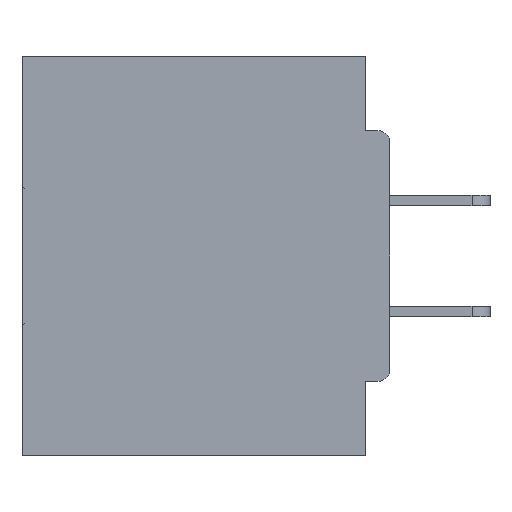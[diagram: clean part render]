
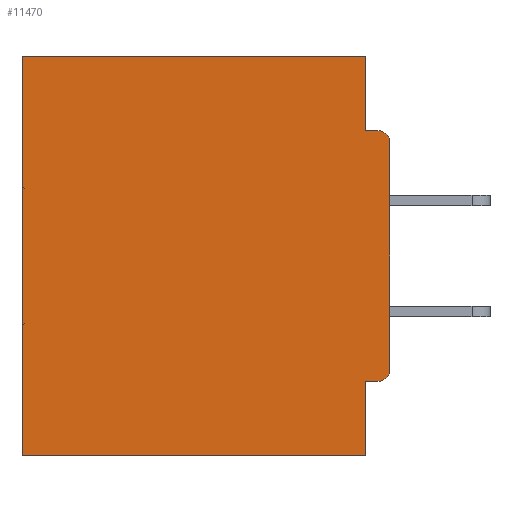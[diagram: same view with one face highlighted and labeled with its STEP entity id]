
A CAD part, left-side view. The second image highlights one B-rep face of the part: STEP entity #11470.
In plain terms, the highlighted planar face has unit normal (-1, 0, 0).
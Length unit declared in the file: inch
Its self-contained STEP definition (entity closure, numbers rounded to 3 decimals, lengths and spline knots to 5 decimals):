
#1285 = LINE ( 'NONE', #10455, #16708 ) ;
#1832 = VECTOR ( 'NONE', #39728, 39.37008 ) ;
#2207 = VERTEX_POINT ( 'NONE', #20075 ) ;
#2713 = LINE ( 'NONE', #6771, #37363 ) ;
#2864 = DIRECTION ( 'NONE',  ( -1., 0., 0. ) ) ;
#3424 = DIRECTION ( 'NONE',  ( 0., 0., -1. ) ) ;
#3531 = VERTEX_POINT ( 'NONE', #36057 ) ;
#3902 = VECTOR ( 'NONE', #17438, 39.37008 ) ;
#3994 = VECTOR ( 'NONE', #11558, 39.37008 ) ;
#5198 = ORIENTED_EDGE ( 'NONE', *, *, #39900, .T. ) ;
#5393 = CARTESIAN_POINT ( 'NONE',  ( 0.298, 0., -0.5 ) ) ;
#5711 = VERTEX_POINT ( 'NONE', #43050 ) ;
#5946 = CARTESIAN_POINT ( 'NONE',  ( 0.298, 0.46, 0. ) ) ;
#6062 = LINE ( 'NONE', #5393, #1832 ) ;
#6728 = EDGE_CURVE ( 'NONE', #20890, #8787, #16250, .T. ) ;
#6771 = CARTESIAN_POINT ( 'NONE',  ( 0.298, 0., -0.4065 ) ) ;
#6812 = VERTEX_POINT ( 'NONE', #8555 ) ;
#7296 = ORIENTED_EDGE ( 'NONE', *, *, #17299, .F. ) ;
#7655 = ORIENTED_EDGE ( 'NONE', *, *, #6728, .T. ) ;
#7831 = CARTESIAN_POINT ( 'NONE',  ( 0.298, 0., 0. ) ) ;
#8555 = CARTESIAN_POINT ( 'NONE',  ( 0.298, 0.46, -0.5 ) ) ;
#8787 = VERTEX_POINT ( 'NONE', #5946 ) ;
#10455 = CARTESIAN_POINT ( 'NONE',  ( 0.298, 0.031, -0.5 ) ) ;
#10601 = CIRCLE ( 'NONE', #30899, 0.015 ) ;
#10845 = ORIENTED_EDGE ( 'NONE', *, *, #43947, .F. ) ;
#11470 = ADVANCED_FACE ( 'NONE', ( #34854 ), #23864, .F. ) ;
#11558 = DIRECTION ( 'NONE',  ( 0., 1., 0. ) ) ;
#11743 = LINE ( 'NONE', #23046, #12156 ) ;
#12156 = VECTOR ( 'NONE', #16825, 39.37008 ) ;
#12641 = ORIENTED_EDGE ( 'NONE', *, *, #33715, .T. ) ;
#13978 = ORIENTED_EDGE ( 'NONE', *, *, #35095, .F. ) ;
#14409 = DIRECTION ( 'NONE',  ( 0., 0., -1. ) ) ;
#16011 = DIRECTION ( 'NONE',  ( 0., 0., -1. ) ) ;
#16181 = ORIENTED_EDGE ( 'NONE', *, *, #34183, .F. ) ;
#16250 = LINE ( 'NONE', #7831, #3994 ) ;
#16550 = VERTEX_POINT ( 'NONE', #39264 ) ;
#16708 = VECTOR ( 'NONE', #37703, 39.37008 ) ;
#16825 = DIRECTION ( 'NONE',  ( 0., 0., -1. ) ) ;
#17299 = EDGE_CURVE ( 'NONE', #5711, #6812, #6062, .T. ) ;
#17438 = DIRECTION ( 'NONE',  ( 0., -1., 0. ) ) ;
#18301 = CARTESIAN_POINT ( 'NONE',  ( 0.298, 0., -0.1085 ) ) ;
#19709 = AXIS2_PLACEMENT_3D ( 'NONE', #39305, #28441, #30352 ) ;
#20075 = CARTESIAN_POINT ( 'NONE',  ( 0.298, 0., -0.3915 ) ) ;
#20427 = CARTESIAN_POINT ( 'NONE',  ( 0.298, 0.031, -0.0935 ) ) ;
#20545 = EDGE_LOOP ( 'NONE', ( #12641, #37215, #16181, #7655, #5198, #7296, #10845, #38088, #25581, #13978 ) ) ;
#20890 = VERTEX_POINT ( 'NONE', #27323 ) ;
#23046 = CARTESIAN_POINT ( 'NONE',  ( 0.298, 0.031, -0.5 ) ) ;
#23247 = CARTESIAN_POINT ( 'NONE',  ( 0.298, 0.015, -0.4065 ) ) ;
#23864 = PLANE ( 'NONE',  #19709 ) ;
#25581 = ORIENTED_EDGE ( 'NONE', *, *, #38496, .T. ) ;
#27323 = CARTESIAN_POINT ( 'NONE',  ( 0.298, 0.031, 0. ) ) ;
#28441 = DIRECTION ( 'NONE',  ( 1., 0., 0. ) ) ;
#28886 = VERTEX_POINT ( 'NONE', #23247 ) ;
#29050 = LINE ( 'NONE', #43078, #38124 ) ;
#29667 = CARTESIAN_POINT ( 'NONE',  ( 0.298, 0.015, -0.1085 ) ) ;
#30352 = DIRECTION ( 'NONE',  ( 0., 0., -1. ) ) ;
#30899 = AXIS2_PLACEMENT_3D ( 'NONE', #37112, #2864, #33693 ) ;
#32700 = EDGE_CURVE ( 'NONE', #40708, #3531, #38495, .T. ) ;
#33204 = EDGE_CURVE ( 'NONE', #28886, #16550, #2713, .T. ) ;
#33693 = DIRECTION ( 'NONE',  ( 0., 0., -1. ) ) ;
#33711 = DIRECTION ( 'NONE',  ( 0., 1., 0. ) ) ;
#33715 = EDGE_CURVE ( 'NONE', #39848, #3531, #41615, .T. ) ;
#34183 = EDGE_CURVE ( 'NONE', #20890, #40708, #11743, .T. ) ;
#34854 = FACE_OUTER_BOUND ( 'NONE', #20545, .T. ) ;
#35095 = EDGE_CURVE ( 'NONE', #39848, #2207, #40332, .T. ) ;
#36057 = CARTESIAN_POINT ( 'NONE',  ( 0.298, 0.015, -0.0935 ) ) ;
#36652 = VECTOR ( 'NONE', #3424, 39.37008 ) ;
#37112 = CARTESIAN_POINT ( 'NONE',  ( 0.298, 0.015, -0.3915 ) ) ;
#37215 = ORIENTED_EDGE ( 'NONE', *, *, #32700, .F. ) ;
#37363 = VECTOR ( 'NONE', #33711, 39.37008 ) ;
#37364 = CARTESIAN_POINT ( 'NONE',  ( 0.298, 0., 0. ) ) ;
#37703 = DIRECTION ( 'NONE',  ( 0., 0., -1. ) ) ;
#38088 = ORIENTED_EDGE ( 'NONE', *, *, #33204, .F. ) ;
#38124 = VECTOR ( 'NONE', #16011, 39.37008 ) ;
#38491 = AXIS2_PLACEMENT_3D ( 'NONE', #29667, #40074, #14409 ) ;
#38495 = LINE ( 'NONE', #40736, #3902 ) ;
#38496 = EDGE_CURVE ( 'NONE', #28886, #2207, #10601, .T. ) ;
#39264 = CARTESIAN_POINT ( 'NONE',  ( 0.298, 0.031, -0.4065 ) ) ;
#39305 = CARTESIAN_POINT ( 'NONE',  ( 0.298, 0., 0. ) ) ;
#39728 = DIRECTION ( 'NONE',  ( 0., 1., 0. ) ) ;
#39848 = VERTEX_POINT ( 'NONE', #18301 ) ;
#39900 = EDGE_CURVE ( 'NONE', #8787, #6812, #29050, .T. ) ;
#40074 = DIRECTION ( 'NONE',  ( -1., 0., 0. ) ) ;
#40332 = LINE ( 'NONE', #37364, #36652 ) ;
#40708 = VERTEX_POINT ( 'NONE', #20427 ) ;
#40736 = CARTESIAN_POINT ( 'NONE',  ( 0.298, 0., -0.0935 ) ) ;
#41615 = CIRCLE ( 'NONE', #38491, 0.015 ) ;
#43050 = CARTESIAN_POINT ( 'NONE',  ( 0.298, 0.031, -0.5 ) ) ;
#43078 = CARTESIAN_POINT ( 'NONE',  ( 0.298, 0.46, 0. ) ) ;
#43947 = EDGE_CURVE ( 'NONE', #16550, #5711, #1285, .T. ) ;
